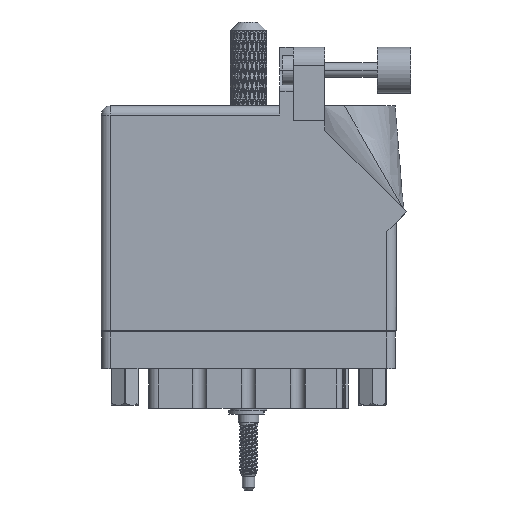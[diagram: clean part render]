
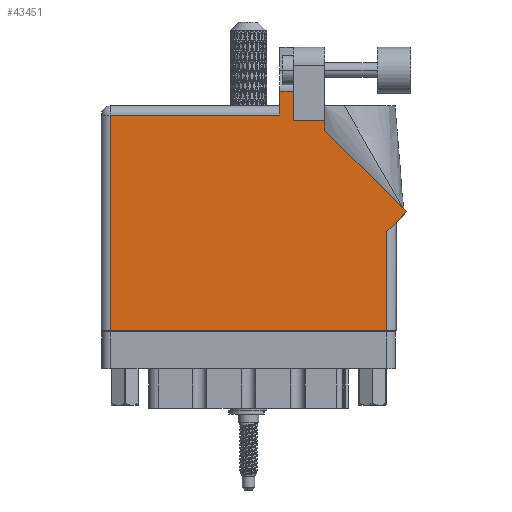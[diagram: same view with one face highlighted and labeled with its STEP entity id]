
A CAD part, front view. The second image highlights one B-rep face of the part: STEP entity #43451.
In plain terms, the highlighted face is planar.
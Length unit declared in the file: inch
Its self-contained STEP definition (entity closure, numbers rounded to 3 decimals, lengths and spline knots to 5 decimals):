
#1478 = EDGE_CURVE ( 'NONE', #19167, #13559, #58420, .T. ) ;
#1641 = EDGE_CURVE ( 'NONE', #11887, #11666, #10715, .T. ) ;
#1988 = VERTEX_POINT ( 'NONE', #64841 ) ;
#2300 = CARTESIAN_POINT ( 'NONE',  ( 2.01, 0.737, 0. ) ) ;
#2481 = DIRECTION ( 'NONE',  ( 1., 0., 0. ) ) ;
#3664 = VECTOR ( 'NONE', #29759, 39.37008 ) ;
#4895 = LINE ( 'NONE', #101977, #58179 ) ;
#9389 = LINE ( 'NONE', #97063, #24785 ) ;
#9710 = DIRECTION ( 'NONE',  ( 0., 1., 0. ) ) ;
#10715 = LINE ( 'NONE', #2300, #3664 ) ;
#11582 = FACE_OUTER_BOUND ( 'NONE', #34545, .T. ) ;
#11666 = VERTEX_POINT ( 'NONE', #38184 ) ;
#11887 = VERTEX_POINT ( 'NONE', #91352 ) ;
#13123 = CARTESIAN_POINT ( 'NONE',  ( 0.062, 1.468, 0. ) ) ;
#13559 = VERTEX_POINT ( 'NONE', #105239 ) ;
#14699 = ORIENTED_EDGE ( 'NONE', *, *, #1478, .T. ) ;
#15116 = ORIENTED_EDGE ( 'NONE', *, *, #26951, .T. ) ;
#16284 = EDGE_CURVE ( 'NONE', #64032, #64134, #26625, .T. ) ;
#16321 = EDGE_CURVE ( 'NONE', #82969, #17615, #70117, .T. ) ;
#17615 = VERTEX_POINT ( 'NONE', #55432 ) ;
#17760 = DIRECTION ( 'NONE',  ( 0., 1., 0. ) ) ;
#18171 = CARTESIAN_POINT ( 'NONE',  ( 1.524, 1.43, 0. ) ) ;
#19016 = VECTOR ( 'NONE', #33773, 39.37008 ) ;
#19167 = VERTEX_POINT ( 'NONE', #47481 ) ;
#20928 = VECTOR ( 'NONE', #43178, 39.37008 ) ;
#23688 = VERTEX_POINT ( 'NONE', #13123 ) ;
#23773 = LINE ( 'NONE', #96811, #20928 ) ;
#24785 = VECTOR ( 'NONE', #106780, 39.37008 ) ;
#25591 = CARTESIAN_POINT ( 'NONE',  ( 1.524, 1.36442, 0. ) ) ;
#26425 = PLANE ( 'NONE',  #48230 ) ;
#26625 = LINE ( 'NONE', #25591, #110653 ) ;
#26951 = EDGE_CURVE ( 'NONE', #13559, #82969, #23773, .T. ) ;
#28664 = DIRECTION ( 'NONE',  ( -1., 0., 0. ) ) ;
#29759 = DIRECTION ( 'NONE',  ( 0.707, 0.707, 0. ) ) ;
#32390 = CARTESIAN_POINT ( 'NONE',  ( 1.524, 1.43, 0. ) ) ;
#32728 = CARTESIAN_POINT ( 'NONE',  ( 1.524, 1.36442, 0. ) ) ;
#33773 = DIRECTION ( 'NONE',  ( 0., 1., 0. ) ) ;
#34268 = CARTESIAN_POINT ( 'NONE',  ( 0.062, 0., 0. ) ) ;
#34545 = EDGE_LOOP ( 'NONE', ( #14699, #15116, #38830, #60103, #55725, #65656, #39526, #64267, #43429, #93290, #90115 ) ) ;
#35336 = LINE ( 'NONE', #32390, #112417 ) ;
#38184 = CARTESIAN_POINT ( 'NONE',  ( 2.08071, 0.80771, 0. ) ) ;
#38830 = ORIENTED_EDGE ( 'NONE', *, *, #16321, .T. ) ;
#39134 = CARTESIAN_POINT ( 'NONE',  ( 2.08071, 0.80771, 0. ) ) ;
#39194 = EDGE_CURVE ( 'NONE', #23688, #52982, #9389, .T. ) ;
#39526 = ORIENTED_EDGE ( 'NONE', *, *, #62821, .T. ) ;
#40835 = EDGE_CURVE ( 'NONE', #52982, #1988, #4895, .T. ) ;
#43178 = DIRECTION ( 'NONE',  ( -1., 0., 0. ) ) ;
#43429 = ORIENTED_EDGE ( 'NONE', *, *, #71509, .T. ) ;
#43451 = ADVANCED_FACE ( 'NONE', ( #11582 ), #26425, .F. ) ;
#44083 = DIRECTION ( 'NONE',  ( 0., -1., 0. ) ) ;
#47481 = CARTESIAN_POINT ( 'NONE',  ( 1.311, 1.43, 0. ) ) ;
#48230 = AXIS2_PLACEMENT_3D ( 'NONE', #107069, #106307, #114933 ) ;
#48432 = VECTOR ( 'NONE', #28664, 39.37008 ) ;
#50482 = VECTOR ( 'NONE', #44083, 39.37008 ) ;
#50658 = LINE ( 'NONE', #99435, #102531 ) ;
#51417 = CARTESIAN_POINT ( 'NONE',  ( 1.311, 1.43, 0. ) ) ;
#52982 = VERTEX_POINT ( 'NONE', #34268 ) ;
#54473 = CARTESIAN_POINT ( 'NONE',  ( 1.217, 1.6315, 0. ) ) ;
#55432 = CARTESIAN_POINT ( 'NONE',  ( 1.217, 1.468, 0. ) ) ;
#55725 = ORIENTED_EDGE ( 'NONE', *, *, #39194, .T. ) ;
#58179 = VECTOR ( 'NONE', #2481, 39.37008 ) ;
#58420 = LINE ( 'NONE', #51417, #19016 ) ;
#60103 = ORIENTED_EDGE ( 'NONE', *, *, #99558, .T. ) ;
#62821 = EDGE_CURVE ( 'NONE', #1988, #11887, #50658, .T. ) ;
#64032 = VERTEX_POINT ( 'NONE', #32728 ) ;
#64134 = VERTEX_POINT ( 'NONE', #18171 ) ;
#64267 = ORIENTED_EDGE ( 'NONE', *, *, #1641, .T. ) ;
#64841 = CARTESIAN_POINT ( 'NONE',  ( 1.948, 0., 0. ) ) ;
#65656 = ORIENTED_EDGE ( 'NONE', *, *, #40835, .T. ) ;
#70117 = LINE ( 'NONE', #116047, #50482 ) ;
#71509 = EDGE_CURVE ( 'NONE', #11666, #64032, #95861, .T. ) ;
#74722 = DIRECTION ( 'NONE',  ( -0.707, 0.707, 0. ) ) ;
#77401 = DIRECTION ( 'NONE',  ( -1., 0., 0. ) ) ;
#82969 = VERTEX_POINT ( 'NONE', #54473 ) ;
#90115 = ORIENTED_EDGE ( 'NONE', *, *, #102067, .T. ) ;
#91352 = CARTESIAN_POINT ( 'NONE',  ( 1.948, 0.675, 0. ) ) ;
#93290 = ORIENTED_EDGE ( 'NONE', *, *, #16284, .T. ) ;
#95861 = LINE ( 'NONE', #39134, #99971 ) ;
#96811 = CARTESIAN_POINT ( 'NONE',  ( 1.64177, 1.6315, 0. ) ) ;
#97063 = CARTESIAN_POINT ( 'NONE',  ( 0.062, 0., 0. ) ) ;
#99435 = CARTESIAN_POINT ( 'NONE',  ( 1.948, 0.737, 0. ) ) ;
#99558 = EDGE_CURVE ( 'NONE', #17615, #23688, #104435, .T. ) ;
#99971 = VECTOR ( 'NONE', #74722, 39.37008 ) ;
#101905 = CARTESIAN_POINT ( 'NONE',  ( 0., 1.468, 0. ) ) ;
#101977 = CARTESIAN_POINT ( 'NONE',  ( 0., 0., 0. ) ) ;
#102067 = EDGE_CURVE ( 'NONE', #64134, #19167, #35336, .T. ) ;
#102531 = VECTOR ( 'NONE', #9710, 39.37008 ) ;
#104435 = LINE ( 'NONE', #101905, #48432 ) ;
#105239 = CARTESIAN_POINT ( 'NONE',  ( 1.311, 1.6315, 0. ) ) ;
#106307 = DIRECTION ( 'NONE',  ( 0., 0., -1. ) ) ;
#106780 = DIRECTION ( 'NONE',  ( 0., -1., 0. ) ) ;
#107069 = CARTESIAN_POINT ( 'NONE',  ( 0., 1.53, 0. ) ) ;
#110653 = VECTOR ( 'NONE', #17760, 39.37008 ) ;
#112417 = VECTOR ( 'NONE', #77401, 39.37008 ) ;
#114933 = DIRECTION ( 'NONE',  ( -1., 0., 0. ) ) ;
#116047 = CARTESIAN_POINT ( 'NONE',  ( 1.217, 1.53, 0. ) ) ;
